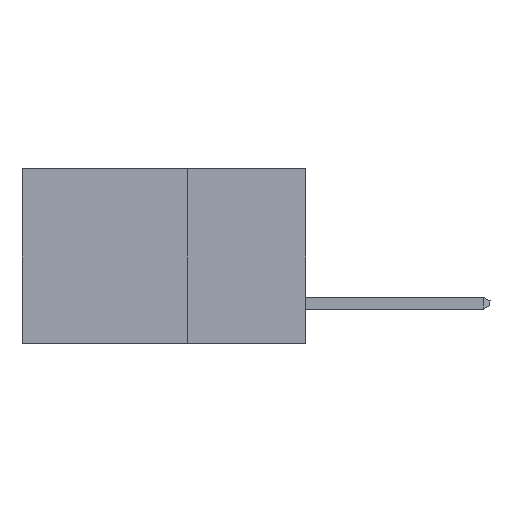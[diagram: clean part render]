
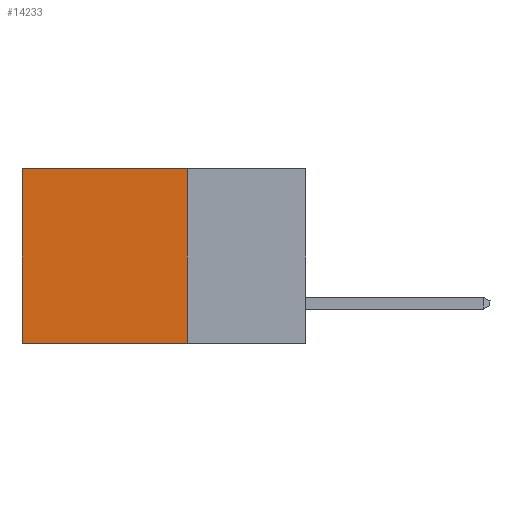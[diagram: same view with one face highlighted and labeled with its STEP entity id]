
A CAD part, left-side view. The second image highlights one B-rep face of the part: STEP entity #14233.
In plain terms, the highlighted planar face has unit normal (-1, 0, 0).
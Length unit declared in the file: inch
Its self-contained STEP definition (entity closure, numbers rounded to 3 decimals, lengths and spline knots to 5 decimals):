
#47 = DIRECTION ( 'NONE',  ( 0., 1., 0. ) ) ;
#261 = CARTESIAN_POINT ( 'NONE',  ( 0.2615, 0.25, -0.37 ) ) ;
#546 = VECTOR ( 'NONE', #14783, 39.37008 ) ;
#913 = LINE ( 'NONE', #10846, #13844 ) ;
#1350 = LINE ( 'NONE', #10978, #4430 ) ;
#2028 = CARTESIAN_POINT ( 'NONE',  ( 0.2615, 0.6, -0.37 ) ) ;
#3762 = EDGE_CURVE ( 'NONE', #20112, #4510, #5279, .T. ) ;
#4430 = VECTOR ( 'NONE', #21245, 39.37008 ) ;
#4501 = CARTESIAN_POINT ( 'NONE',  ( 0.2615, 0.25, -0.37 ) ) ;
#4510 = VERTEX_POINT ( 'NONE', #2028 ) ;
#5279 = LINE ( 'NONE', #11933, #546 ) ;
#6025 = EDGE_CURVE ( 'NONE', #11856, #4510, #18192, .T. ) ;
#6335 = FACE_OUTER_BOUND ( 'NONE', #18863, .T. ) ;
#6349 = ORIENTED_EDGE ( 'NONE', *, *, #3762, .T. ) ;
#6487 = VECTOR ( 'NONE', #47, 39.37008 ) ;
#6904 = ORIENTED_EDGE ( 'NONE', *, *, #12256, .F. ) ;
#7392 = CARTESIAN_POINT ( 'NONE',  ( 0.2615, 0.6, 0. ) ) ;
#8076 = DIRECTION ( 'NONE',  ( 0., 0., -1. ) ) ;
#9003 = AXIS2_PLACEMENT_3D ( 'NONE', #4501, #16288, #8076 ) ;
#10846 = CARTESIAN_POINT ( 'NONE',  ( 0.2615, 0.25, 0. ) ) ;
#10978 = CARTESIAN_POINT ( 'NONE',  ( 0.2615, 0.25, -0.37 ) ) ;
#11856 = VERTEX_POINT ( 'NONE', #17782 ) ;
#11933 = CARTESIAN_POINT ( 'NONE',  ( 0.2615, 0.6, -0.37 ) ) ;
#12256 = EDGE_CURVE ( 'NONE', #12612, #11856, #1350, .T. ) ;
#12272 = DIRECTION ( 'NONE',  ( 0., 1., 0. ) ) ;
#12612 = VERTEX_POINT ( 'NONE', #19083 ) ;
#13844 = VECTOR ( 'NONE', #12272, 39.37008 ) ;
#14233 = ADVANCED_FACE ( 'NONE', ( #6335 ), #19445, .F. ) ;
#14783 = DIRECTION ( 'NONE',  ( 0., 0., -1. ) ) ;
#14879 = EDGE_CURVE ( 'NONE', #12612, #20112, #913, .T. ) ;
#15489 = ORIENTED_EDGE ( 'NONE', *, *, #6025, .F. ) ;
#16288 = DIRECTION ( 'NONE',  ( 1., 0., 0. ) ) ;
#17614 = ORIENTED_EDGE ( 'NONE', *, *, #14879, .T. ) ;
#17782 = CARTESIAN_POINT ( 'NONE',  ( 0.2615, 0.25, -0.37 ) ) ;
#18192 = LINE ( 'NONE', #261, #6487 ) ;
#18863 = EDGE_LOOP ( 'NONE', ( #6349, #15489, #6904, #17614 ) ) ;
#19083 = CARTESIAN_POINT ( 'NONE',  ( 0.2615, 0.25, 0. ) ) ;
#19445 = PLANE ( 'NONE',  #9003 ) ;
#20112 = VERTEX_POINT ( 'NONE', #7392 ) ;
#21245 = DIRECTION ( 'NONE',  ( 0., 0., -1. ) ) ;
